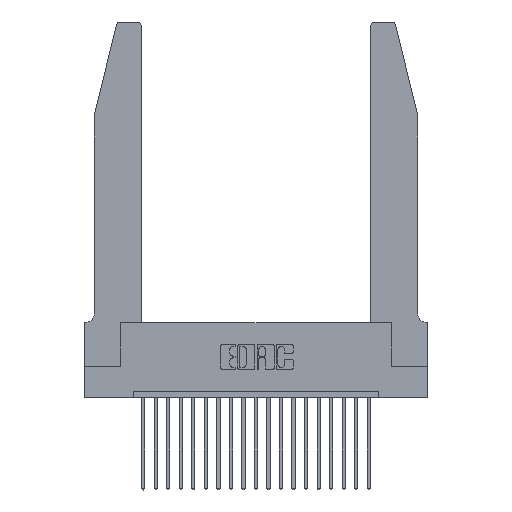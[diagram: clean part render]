
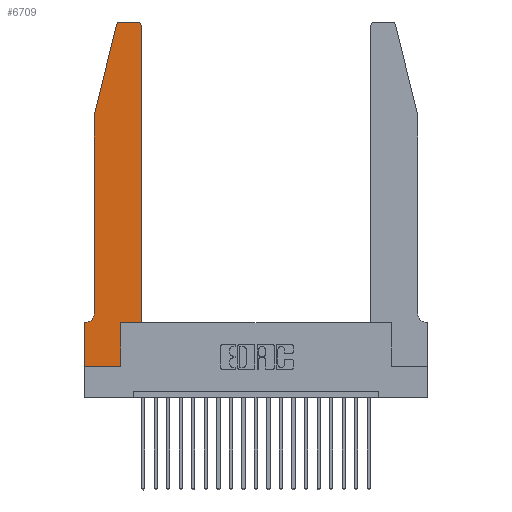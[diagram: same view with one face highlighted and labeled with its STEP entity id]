
A CAD part, top view. The second image highlights one B-rep face of the part: STEP entity #6709.
In plain terms, the highlighted planar face has unit normal (0, 0, 1).
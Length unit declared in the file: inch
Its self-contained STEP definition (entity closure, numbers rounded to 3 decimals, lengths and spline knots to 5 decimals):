
#69 = VECTOR ( 'NONE', #12929, 39.37008 ) ;
#260 = CARTESIAN_POINT ( 'NONE',  ( 0.4205, 2.75, 0.37 ) ) ;
#261 = DIRECTION ( 'NONE',  ( -1., 0., 0. ) ) ;
#462 = DIRECTION ( 'NONE',  ( 1., 0., 0. ) ) ;
#834 = VERTEX_POINT ( 'NONE', #21131 ) ;
#1155 = LINE ( 'NONE', #19721, #69 ) ;
#1156 = DIRECTION ( 'NONE',  ( -0.239, -0.971, 0. ) ) ;
#1222 = CARTESIAN_POINT ( 'NONE',  ( 0.0755, 0.42, 0.37 ) ) ;
#1240 = VERTEX_POINT ( 'NONE', #260 ) ;
#1653 = EDGE_CURVE ( 'NONE', #18147, #834, #2835, .T. ) ;
#1912 = VERTEX_POINT ( 'NONE', #10425 ) ;
#2046 = CARTESIAN_POINT ( 'NONE',  ( 0.284, 2.75, 0.37 ) ) ;
#2414 = VECTOR ( 'NONE', #19120, 39.37008 ) ;
#2802 = VERTEX_POINT ( 'NONE', #1222 ) ;
#2820 = CARTESIAN_POINT ( 'NONE',  ( 0.0055, 0.35, 0.37 ) ) ;
#2835 = LINE ( 'NONE', #17874, #16178 ) ;
#3090 = ORIENTED_EDGE ( 'NONE', *, *, #11733, .T. ) ;
#3331 = CARTESIAN_POINT ( 'NONE',  ( 0.2865, 0., 0.37 ) ) ;
#3555 = CARTESIAN_POINT ( 'NONE',  ( 0., 0., 0.37 ) ) ;
#3886 = EDGE_CURVE ( 'NONE', #1240, #19367, #7598, .T. ) ;
#4430 = DIRECTION ( 'NONE',  ( 1., 0., 0. ) ) ;
#4966 = EDGE_CURVE ( 'NONE', #21797, #8055, #18495, .T. ) ;
#4974 = CIRCLE ( 'NONE', #14974, 0.03 ) ;
#6087 = VECTOR ( 'NONE', #13395, 39.37008 ) ;
#6343 = CARTESIAN_POINT ( 'NONE',  ( 0.2605, 2.75, 0.37 ) ) ;
#6444 = LINE ( 'NONE', #19320, #2414 ) ;
#6537 = CARTESIAN_POINT ( 'NONE',  ( 0.4505, 2.72, 0.37 ) ) ;
#6709 = ADVANCED_FACE ( 'NONE', ( #9645 ), #19225, .T. ) ;
#6976 = ORIENTED_EDGE ( 'NONE', *, *, #17231, .T. ) ;
#7010 = AXIS2_PLACEMENT_3D ( 'NONE', #10330, #13545, #18754 ) ;
#7384 = VERTEX_POINT ( 'NONE', #6537 ) ;
#7590 = DIRECTION ( 'NONE',  ( 1., 0., 0. ) ) ;
#7598 = LINE ( 'NONE', #6343, #18281 ) ;
#7663 = VECTOR ( 'NONE', #261, 39.37008 ) ;
#7737 = ORIENTED_EDGE ( 'NONE', *, *, #13914, .T. ) ;
#8055 = VERTEX_POINT ( 'NONE', #3331 ) ;
#8237 = EDGE_CURVE ( 'NONE', #8055, #18147, #19969, .T. ) ;
#8355 = VECTOR ( 'NONE', #17841, 39.37008 ) ;
#8796 = DIRECTION ( 'NONE',  ( 0., 0., 1. ) ) ;
#8950 = CARTESIAN_POINT ( 'NONE',  ( 0.0755, 0.35, 0.37 ) ) ;
#9067 = EDGE_CURVE ( 'NONE', #10257, #1912, #19665, .T. ) ;
#9208 = VECTOR ( 'NONE', #1156, 39.37008 ) ;
#9645 = FACE_OUTER_BOUND ( 'NONE', #13602, .T. ) ;
#9769 = EDGE_CURVE ( 'NONE', #19367, #12238, #4974, .T. ) ;
#9793 = DIRECTION ( 'NONE',  ( 0., 1., 0. ) ) ;
#10257 = VERTEX_POINT ( 'NONE', #2820 ) ;
#10330 = CARTESIAN_POINT ( 'NONE',  ( 0.4205, 2.72, 0.37 ) ) ;
#10425 = CARTESIAN_POINT ( 'NONE',  ( 0., 0.35, 0.37 ) ) ;
#10840 = CARTESIAN_POINT ( 'NONE',  ( 0., 0., 0.37 ) ) ;
#11237 = ORIENTED_EDGE ( 'NONE', *, *, #4966, .T. ) ;
#11733 = EDGE_CURVE ( 'NONE', #7384, #1240, #17158, .T. ) ;
#12238 = VERTEX_POINT ( 'NONE', #21353 ) ;
#12713 = CARTESIAN_POINT ( 'NONE',  ( 0.2865, 0.35, 0.37 ) ) ;
#12831 = LINE ( 'NONE', #20229, #17106 ) ;
#12929 = DIRECTION ( 'NONE',  ( 0., -1., 0. ) ) ;
#13395 = DIRECTION ( 'NONE',  ( 0., 1., 0. ) ) ;
#13545 = DIRECTION ( 'NONE',  ( 0., 0., 1. ) ) ;
#13602 = EDGE_LOOP ( 'NONE', ( #18820, #17547, #6976, #19357, #17954, #14204, #7737, #11237, #18781, #21201, #18479, #3090 ) ) ;
#13914 = EDGE_CURVE ( 'NONE', #1912, #21797, #6444, .T. ) ;
#14184 = EDGE_CURVE ( 'NONE', #834, #7384, #12831, .T. ) ;
#14204 = ORIENTED_EDGE ( 'NONE', *, *, #9067, .T. ) ;
#14974 = AXIS2_PLACEMENT_3D ( 'NONE', #19509, #18009, #4430 ) ;
#15110 = DIRECTION ( 'NONE',  ( 0., 0., -1. ) ) ;
#15364 = AXIS2_PLACEMENT_3D ( 'NONE', #21918, #15110, #22147 ) ;
#16178 = VECTOR ( 'NONE', #7590, 39.37008 ) ;
#16943 = AXIS2_PLACEMENT_3D ( 'NONE', #19014, #8796, #462 ) ;
#17106 = VECTOR ( 'NONE', #9793, 39.37008 ) ;
#17158 = CIRCLE ( 'NONE', #7010, 0.03 ) ;
#17231 = EDGE_CURVE ( 'NONE', #12238, #20883, #21765, .T. ) ;
#17547 = ORIENTED_EDGE ( 'NONE', *, *, #9769, .T. ) ;
#17841 = DIRECTION ( 'NONE',  ( 1., 0., 0. ) ) ;
#17874 = CARTESIAN_POINT ( 'NONE',  ( 0.4505, 0.35, 0.37 ) ) ;
#17954 = ORIENTED_EDGE ( 'NONE', *, *, #19396, .T. ) ;
#18009 = DIRECTION ( 'NONE',  ( 0., 0., 1. ) ) ;
#18147 = VERTEX_POINT ( 'NONE', #12713 ) ;
#18262 = EDGE_CURVE ( 'NONE', #20883, #2802, #1155, .T. ) ;
#18281 = VECTOR ( 'NONE', #21793, 39.37008 ) ;
#18469 = CARTESIAN_POINT ( 'NONE',  ( 0.2865, 0.35, 0.37 ) ) ;
#18479 = ORIENTED_EDGE ( 'NONE', *, *, #14184, .T. ) ;
#18495 = LINE ( 'NONE', #10840, #8355 ) ;
#18754 = DIRECTION ( 'NONE',  ( 1., 0., 0. ) ) ;
#18781 = ORIENTED_EDGE ( 'NONE', *, *, #8237, .T. ) ;
#18820 = ORIENTED_EDGE ( 'NONE', *, *, #3886, .T. ) ;
#19014 = CARTESIAN_POINT ( 'NONE',  ( 0., 0.35, 0.37 ) ) ;
#19095 = CIRCLE ( 'NONE', #15364, 0.07 ) ;
#19120 = DIRECTION ( 'NONE',  ( 0., -1., 0. ) ) ;
#19225 = PLANE ( 'NONE',  #16943 ) ;
#19320 = CARTESIAN_POINT ( 'NONE',  ( 0., 0., 0.37 ) ) ;
#19357 = ORIENTED_EDGE ( 'NONE', *, *, #18262, .T. ) ;
#19367 = VERTEX_POINT ( 'NONE', #2046 ) ;
#19396 = EDGE_CURVE ( 'NONE', #2802, #10257, #19095, .T. ) ;
#19509 = CARTESIAN_POINT ( 'NONE',  ( 0.284, 2.72, 0.37 ) ) ;
#19665 = LINE ( 'NONE', #8950, #7663 ) ;
#19721 = CARTESIAN_POINT ( 'NONE',  ( 0.0755, 2., 0.37 ) ) ;
#19969 = LINE ( 'NONE', #18469, #6087 ) ;
#19990 = CARTESIAN_POINT ( 'NONE',  ( 0.0755, 2., 0.37 ) ) ;
#20229 = CARTESIAN_POINT ( 'NONE',  ( 0.4505, 0.35, 0.37 ) ) ;
#20883 = VERTEX_POINT ( 'NONE', #21247 ) ;
#21131 = CARTESIAN_POINT ( 'NONE',  ( 0.4505, 0.35, 0.37 ) ) ;
#21201 = ORIENTED_EDGE ( 'NONE', *, *, #1653, .T. ) ;
#21247 = CARTESIAN_POINT ( 'NONE',  ( 0.0755, 2., 0.37 ) ) ;
#21353 = CARTESIAN_POINT ( 'NONE',  ( 0.25487, 2.72718, 0.37 ) ) ;
#21765 = LINE ( 'NONE', #19990, #9208 ) ;
#21793 = DIRECTION ( 'NONE',  ( -1., 0., 0. ) ) ;
#21797 = VERTEX_POINT ( 'NONE', #3555 ) ;
#21918 = CARTESIAN_POINT ( 'NONE',  ( 0.0055, 0.42, 0.37 ) ) ;
#22147 = DIRECTION ( 'NONE',  ( -1., 0., 0. ) ) ;
